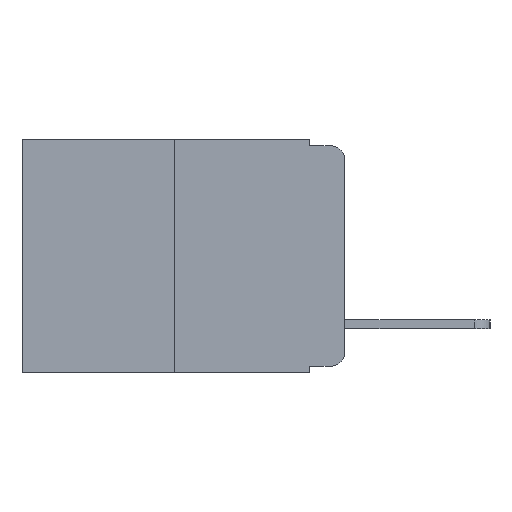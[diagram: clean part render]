
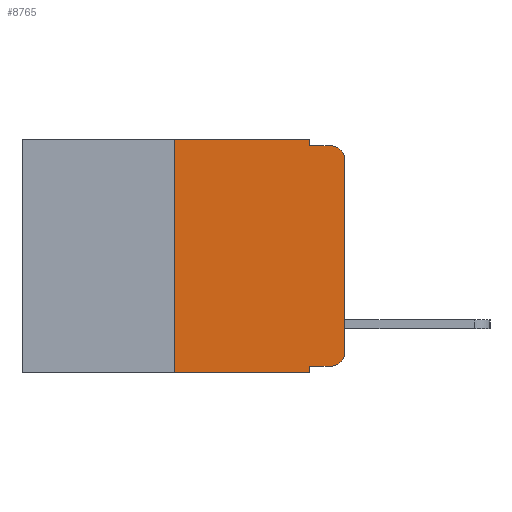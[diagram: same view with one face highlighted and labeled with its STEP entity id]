
A CAD part, left-side view. The second image highlights one B-rep face of the part: STEP entity #8765.
In plain terms, the highlighted planar face has unit normal (-1, 0, 0).
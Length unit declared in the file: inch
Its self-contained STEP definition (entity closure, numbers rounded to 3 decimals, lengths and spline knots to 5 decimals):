
#195 = CARTESIAN_POINT ( 'NONE',  ( 0., 0., 0. ) ) ;
#369 = DIRECTION ( 'NONE',  ( 0., 0., -1. ) ) ;
#629 = VECTOR ( 'NONE', #3035, 39.37008 ) ;
#1176 = EDGE_CURVE ( 'NONE', #3045, #10359, #12155, .T. ) ;
#1326 = EDGE_CURVE ( 'NONE', #14629, #7039, #16439, .T. ) ;
#1573 = EDGE_CURVE ( 'NONE', #6300, #11564, #15642, .T. ) ;
#2148 = EDGE_CURVE ( 'NONE', #6824, #11564, #3305, .T. ) ;
#2343 = CARTESIAN_POINT ( 'NONE',  ( 0., 0.051, 0. ) ) ;
#2501 = EDGE_CURVE ( 'NONE', #9619, #6300, #5540, .T. ) ;
#2591 = LINE ( 'NONE', #4685, #5937 ) ;
#2719 = CARTESIAN_POINT ( 'NONE',  ( 0., 0.051, 0. ) ) ;
#3035 = DIRECTION ( 'NONE',  ( 0., 0., 1. ) ) ;
#3045 = VERTEX_POINT ( 'NONE', #3916 ) ;
#3091 = EDGE_CURVE ( 'NONE', #16464, #6824, #8839, .T. ) ;
#3285 = VECTOR ( 'NONE', #3358, 39.37008 ) ;
#3305 = LINE ( 'NONE', #14346, #14086 ) ;
#3358 = DIRECTION ( 'NONE',  ( 0., -1., 0. ) ) ;
#3916 = CARTESIAN_POINT ( 'NONE',  ( 0., 0.25, -0.343 ) ) ;
#4194 = ORIENTED_EDGE ( 'NONE', *, *, #1573, .T. ) ;
#4350 = ORIENTED_EDGE ( 'NONE', *, *, #2501, .T. ) ;
#4374 = ORIENTED_EDGE ( 'NONE', *, *, #2148, .F. ) ;
#4427 = ORIENTED_EDGE ( 'NONE', *, *, #3091, .F. ) ;
#4461 = CARTESIAN_POINT ( 'NONE',  ( 0., 0.25, 0. ) ) ;
#4474 = ORIENTED_EDGE ( 'NONE', *, *, #15138, .F. ) ;
#4487 = CARTESIAN_POINT ( 'NONE',  ( 0., 0.051, 0. ) ) ;
#4685 = CARTESIAN_POINT ( 'NONE',  ( 0., 0.051, -0.333 ) ) ;
#4689 = ORIENTED_EDGE ( 'NONE', *, *, #1176, .F. ) ;
#4714 = CARTESIAN_POINT ( 'NONE',  ( 0., 0.051, -0.343 ) ) ;
#4874 = ORIENTED_EDGE ( 'NONE', *, *, #10368, .T. ) ;
#4888 = ORIENTED_EDGE ( 'NONE', *, *, #1326, .F. ) ;
#4921 = ORIENTED_EDGE ( 'NONE', *, *, #12741, .T. ) ;
#4983 = ORIENTED_EDGE ( 'NONE', *, *, #9803, .T. ) ;
#5101 = VECTOR ( 'NONE', #9378, 39.37008 ) ;
#5218 = CARTESIAN_POINT ( 'NONE',  ( 0., 0.051, -0.333 ) ) ;
#5473 = DIRECTION ( 'NONE',  ( 0., -1., 0. ) ) ;
#5512 = CARTESIAN_POINT ( 'NONE',  ( 0., 0.02, -0.313 ) ) ;
#5540 = LINE ( 'NONE', #195, #11888 ) ;
#5937 = VECTOR ( 'NONE', #6098, 39.37008 ) ;
#6021 = VECTOR ( 'NONE', #17151, 39.37008 ) ;
#6098 = DIRECTION ( 'NONE',  ( 0., -1., 0. ) ) ;
#6140 = CARTESIAN_POINT ( 'NONE',  ( 0., 0.473, 0. ) ) ;
#6300 = VERTEX_POINT ( 'NONE', #6779 ) ;
#6713 = CIRCLE ( 'NONE', #7801, 0.02 ) ;
#6779 = CARTESIAN_POINT ( 'NONE',  ( 0., 0., -0.03 ) ) ;
#6824 = VERTEX_POINT ( 'NONE', #16201 ) ;
#6904 = DIRECTION ( 'NONE',  ( 0., 0., -1. ) ) ;
#7022 = CARTESIAN_POINT ( 'NONE',  ( 0., 0.02, -0.333 ) ) ;
#7039 = VERTEX_POINT ( 'NONE', #4714 ) ;
#7326 = CARTESIAN_POINT ( 'NONE',  ( 0., 0.473, -0.343 ) ) ;
#7452 = LINE ( 'NONE', #7326, #17263 ) ;
#7801 = AXIS2_PLACEMENT_3D ( 'NONE', #5512, #14799, #6904 ) ;
#8201 = FACE_OUTER_BOUND ( 'NONE', #15805, .T. ) ;
#8496 = AXIS2_PLACEMENT_3D ( 'NONE', #17344, #8699, #15742 ) ;
#8699 = DIRECTION ( 'NONE',  ( -1., 0., 0. ) ) ;
#8765 = ADVANCED_FACE ( 'NONE', ( #8201 ), #16563, .F. ) ;
#8839 = LINE ( 'NONE', #4487, #5101 ) ;
#8967 = DIRECTION ( 'NONE',  ( 1., 0., 0. ) ) ;
#9378 = DIRECTION ( 'NONE',  ( 0., 0., -1. ) ) ;
#9567 = VERTEX_POINT ( 'NONE', #7022 ) ;
#9619 = VERTEX_POINT ( 'NONE', #13745 ) ;
#9803 = EDGE_CURVE ( 'NONE', #14629, #9567, #2591, .T. ) ;
#10155 = CARTESIAN_POINT ( 'NONE',  ( 0., 0.25, 0. ) ) ;
#10359 = VERTEX_POINT ( 'NONE', #4461 ) ;
#10368 = EDGE_CURVE ( 'NONE', #3045, #7039, #7452, .T. ) ;
#11564 = VERTEX_POINT ( 'NONE', #12476 ) ;
#11888 = VECTOR ( 'NONE', #14078, 39.37008 ) ;
#12155 = LINE ( 'NONE', #10155, #629 ) ;
#12476 = CARTESIAN_POINT ( 'NONE',  ( 0., 0.02, -0.01 ) ) ;
#12741 = EDGE_CURVE ( 'NONE', #9567, #9619, #6713, .T. ) ;
#12909 = CARTESIAN_POINT ( 'NONE',  ( 0., 0.473, 0. ) ) ;
#13745 = CARTESIAN_POINT ( 'NONE',  ( 0., 0., -0.313 ) ) ;
#13787 = AXIS2_PLACEMENT_3D ( 'NONE', #6140, #8967, #369 ) ;
#14076 = LINE ( 'NONE', #12909, #3285 ) ;
#14078 = DIRECTION ( 'NONE',  ( 0., 0., 1. ) ) ;
#14086 = VECTOR ( 'NONE', #5473, 39.37008 ) ;
#14346 = CARTESIAN_POINT ( 'NONE',  ( 0., 0.051, -0.01 ) ) ;
#14629 = VERTEX_POINT ( 'NONE', #5218 ) ;
#14799 = DIRECTION ( 'NONE',  ( -1., 0., 0. ) ) ;
#15138 = EDGE_CURVE ( 'NONE', #10359, #16464, #14076, .T. ) ;
#15642 = CIRCLE ( 'NONE', #8496, 0.02 ) ;
#15742 = DIRECTION ( 'NONE',  ( 0., 0., -1. ) ) ;
#15805 = EDGE_LOOP ( 'NONE', ( #4350, #4194, #4374, #4427, #4474, #4689, #4874, #4888, #4983, #4921 ) ) ;
#16201 = CARTESIAN_POINT ( 'NONE',  ( 0., 0.051, -0.01 ) ) ;
#16363 = DIRECTION ( 'NONE',  ( 0., -1., 0. ) ) ;
#16439 = LINE ( 'NONE', #2343, #6021 ) ;
#16464 = VERTEX_POINT ( 'NONE', #2719 ) ;
#16563 = PLANE ( 'NONE',  #13787 ) ;
#17151 = DIRECTION ( 'NONE',  ( 0., 0., -1. ) ) ;
#17263 = VECTOR ( 'NONE', #16363, 39.37008 ) ;
#17344 = CARTESIAN_POINT ( 'NONE',  ( 0., 0.02, -0.03 ) ) ;
